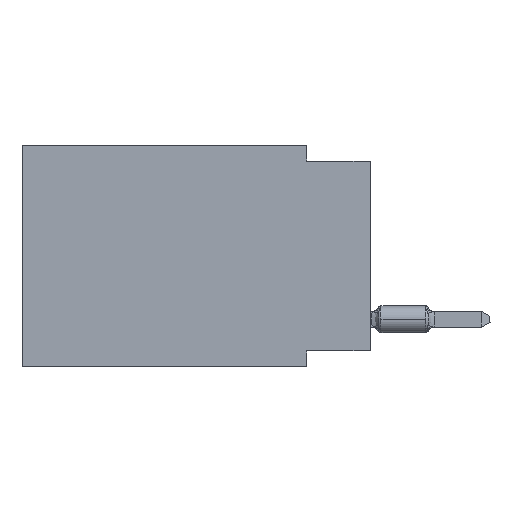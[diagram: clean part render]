
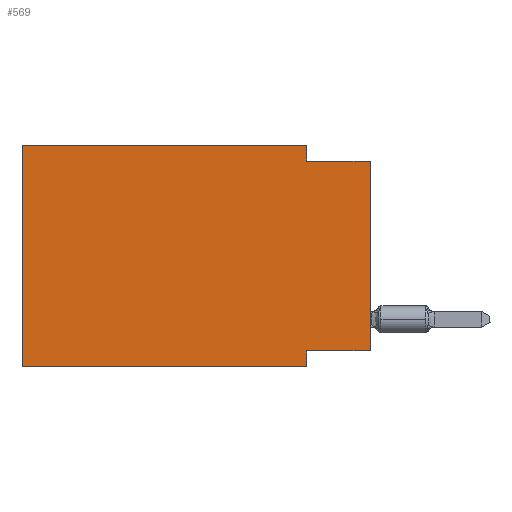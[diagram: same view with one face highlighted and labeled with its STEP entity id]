
A CAD part, left-side view. The second image highlights one B-rep face of the part: STEP entity #569.
In plain terms, the highlighted planar face has unit normal (-1, 0, 0).
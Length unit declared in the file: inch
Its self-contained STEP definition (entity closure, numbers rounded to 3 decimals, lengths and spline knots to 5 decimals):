
#201 = CARTESIAN_POINT ( 'NONE',  ( 0., 0.1, 0. ) ) ;
#283 = LINE ( 'NONE', #26129, #37057 ) ;
#569 = ADVANCED_FACE ( 'NONE', ( #18510 ), #9744, .F. ) ;
#1442 = AXIS2_PLACEMENT_3D ( 'NONE', #15678, #37624, #24889 ) ;
#2813 = VECTOR ( 'NONE', #7354, 39.37008 ) ;
#3412 = CARTESIAN_POINT ( 'NONE',  ( 0., 0.1, -0.35 ) ) ;
#3434 = VERTEX_POINT ( 'NONE', #10998 ) ;
#3465 = CARTESIAN_POINT ( 'NONE',  ( 0., 0., -0.325 ) ) ;
#3870 = CARTESIAN_POINT ( 'NONE',  ( 0., 0., 0. ) ) ;
#4112 = ORIENTED_EDGE ( 'NONE', *, *, #6612, .T. ) ;
#5361 = VECTOR ( 'NONE', #13900, 39.37008 ) ;
#6123 = LINE ( 'NONE', #22745, #2813 ) ;
#6218 = VERTEX_POINT ( 'NONE', #8198 ) ;
#6612 = EDGE_CURVE ( 'NONE', #37921, #12547, #36859, .T. ) ;
#7354 = DIRECTION ( 'NONE',  ( 0., 0., -1. ) ) ;
#7457 = ORIENTED_EDGE ( 'NONE', *, *, #29605, .F. ) ;
#8198 = CARTESIAN_POINT ( 'NONE',  ( 0., 0.55, 0. ) ) ;
#9744 = PLANE ( 'NONE',  #1442 ) ;
#10989 = ORIENTED_EDGE ( 'NONE', *, *, #15313, .F. ) ;
#10998 = CARTESIAN_POINT ( 'NONE',  ( 0., 0., -0.025 ) ) ;
#11098 = VERTEX_POINT ( 'NONE', #3465 ) ;
#12547 = VERTEX_POINT ( 'NONE', #3412 ) ;
#13900 = DIRECTION ( 'NONE',  ( 0., 0., -1. ) ) ;
#14801 = VECTOR ( 'NONE', #27778, 39.37008 ) ;
#14810 = LINE ( 'NONE', #17761, #24494 ) ;
#15313 = EDGE_CURVE ( 'NONE', #27365, #12547, #21754, .T. ) ;
#15678 = CARTESIAN_POINT ( 'NONE',  ( 0., 0.55, 0. ) ) ;
#15980 = ORIENTED_EDGE ( 'NONE', *, *, #32472, .F. ) ;
#16081 = CARTESIAN_POINT ( 'NONE',  ( 0., 0.55, -0.35 ) ) ;
#17043 = EDGE_CURVE ( 'NONE', #11098, #27365, #14810, .T. ) ;
#17448 = DIRECTION ( 'NONE',  ( 0., -1., 0. ) ) ;
#17761 = CARTESIAN_POINT ( 'NONE',  ( 0., 0., -0.325 ) ) ;
#18510 = FACE_OUTER_BOUND ( 'NONE', #39401, .T. ) ;
#18513 = ORIENTED_EDGE ( 'NONE', *, *, #36018, .F. ) ;
#18663 = CARTESIAN_POINT ( 'NONE',  ( 0., 0., -0.025 ) ) ;
#21754 = LINE ( 'NONE', #32321, #5361 ) ;
#22745 = CARTESIAN_POINT ( 'NONE',  ( 0., 0.1, 0. ) ) ;
#23436 = ORIENTED_EDGE ( 'NONE', *, *, #17043, .F. ) ;
#24447 = VECTOR ( 'NONE', #31691, 39.37008 ) ;
#24494 = VECTOR ( 'NONE', #33089, 39.37008 ) ;
#24889 = DIRECTION ( 'NONE',  ( 0., 0., -1. ) ) ;
#25697 = VECTOR ( 'NONE', #17448, 39.37008 ) ;
#26129 = CARTESIAN_POINT ( 'NONE',  ( 0., 0.55, 0. ) ) ;
#27016 = VERTEX_POINT ( 'NONE', #201 ) ;
#27365 = VERTEX_POINT ( 'NONE', #31576 ) ;
#27778 = DIRECTION ( 'NONE',  ( 0., -1., 0. ) ) ;
#29016 = CARTESIAN_POINT ( 'NONE',  ( 0., 0.55, -0.35 ) ) ;
#29605 = EDGE_CURVE ( 'NONE', #27016, #30815, #6123, .T. ) ;
#29809 = LINE ( 'NONE', #34678, #24447 ) ;
#30815 = VERTEX_POINT ( 'NONE', #35313 ) ;
#31124 = ORIENTED_EDGE ( 'NONE', *, *, #33226, .T. ) ;
#31425 = DIRECTION ( 'NONE',  ( 0., 0., 1. ) ) ;
#31576 = CARTESIAN_POINT ( 'NONE',  ( 0., 0.1, -0.325 ) ) ;
#31691 = DIRECTION ( 'NONE',  ( 0., 0., 1. ) ) ;
#32321 = CARTESIAN_POINT ( 'NONE',  ( 0., 0.1, -0.35 ) ) ;
#32472 = EDGE_CURVE ( 'NONE', #30815, #3434, #38543, .T. ) ;
#33089 = DIRECTION ( 'NONE',  ( 0., 1., 0. ) ) ;
#33226 = EDGE_CURVE ( 'NONE', #11098, #3434, #37786, .T. ) ;
#34678 = CARTESIAN_POINT ( 'NONE',  ( 0., 0.55, 0. ) ) ;
#35313 = CARTESIAN_POINT ( 'NONE',  ( 0., 0.1, -0.025 ) ) ;
#35374 = VECTOR ( 'NONE', #31425, 39.37008 ) ;
#36018 = EDGE_CURVE ( 'NONE', #37921, #6218, #29809, .T. ) ;
#36105 = EDGE_CURVE ( 'NONE', #6218, #27016, #283, .T. ) ;
#36859 = LINE ( 'NONE', #29016, #25697 ) ;
#37057 = VECTOR ( 'NONE', #38038, 39.37008 ) ;
#37624 = DIRECTION ( 'NONE',  ( 1., 0., 0. ) ) ;
#37786 = LINE ( 'NONE', #3870, #35374 ) ;
#37921 = VERTEX_POINT ( 'NONE', #16081 ) ;
#38038 = DIRECTION ( 'NONE',  ( 0., -1., 0. ) ) ;
#38543 = LINE ( 'NONE', #18663, #14801 ) ;
#39214 = ORIENTED_EDGE ( 'NONE', *, *, #36105, .F. ) ;
#39401 = EDGE_LOOP ( 'NONE', ( #31124, #15980, #7457, #39214, #18513, #4112, #10989, #23436 ) ) ;
